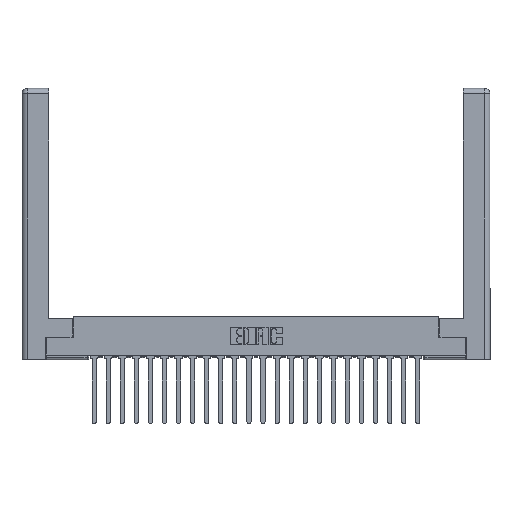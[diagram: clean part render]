
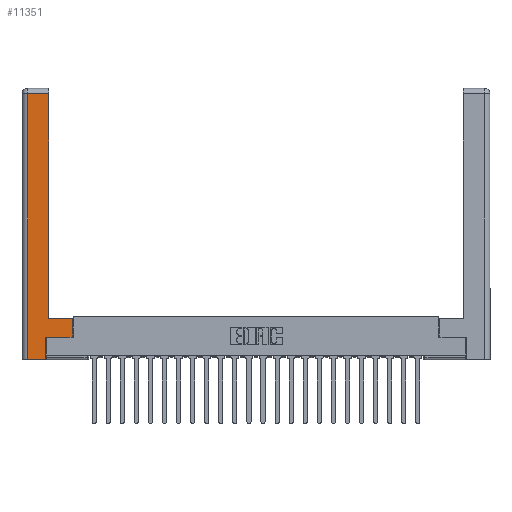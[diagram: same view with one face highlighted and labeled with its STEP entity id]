
A CAD part, top view. The second image highlights one B-rep face of the part: STEP entity #11351.
In plain terms, the highlighted planar face has unit normal (0, 0, 1).
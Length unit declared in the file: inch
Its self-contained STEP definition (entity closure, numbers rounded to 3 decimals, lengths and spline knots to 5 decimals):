
#398 = LINE ( 'NONE', #23268, #8163 ) ;
#634 = LINE ( 'NONE', #24262, #15480 ) ;
#1180 = ORIENTED_EDGE ( 'NONE', *, *, #20733, .T. ) ;
#2334 = CARTESIAN_POINT ( 'NONE',  ( 0.0615, 0., 0. ) ) ;
#2374 = EDGE_CURVE ( 'NONE', #14842, #12267, #24141, .T. ) ;
#2509 = CARTESIAN_POINT ( 'NONE',  ( 0.0615, 2.94, 0. ) ) ;
#2754 = DIRECTION ( 'NONE',  ( 0., 1., 0. ) ) ;
#2984 = CARTESIAN_POINT ( 'NONE',  ( 0.565, 0.45, 0. ) ) ;
#3222 = DIRECTION ( 'NONE',  ( -1., 0., 0. ) ) ;
#3646 = EDGE_CURVE ( 'NONE', #18784, #19529, #634, .T. ) ;
#4583 = CARTESIAN_POINT ( 'NONE',  ( 0.0615, 0., 0. ) ) ;
#5269 = CARTESIAN_POINT ( 'NONE',  ( 0.265, 0., 0. ) ) ;
#5600 = ORIENTED_EDGE ( 'NONE', *, *, #18948, .T. ) ;
#5623 = ORIENTED_EDGE ( 'NONE', *, *, #21719, .T. ) ;
#5715 = DIRECTION ( 'NONE',  ( -1., 0., 0. ) ) ;
#6089 = EDGE_CURVE ( 'NONE', #19529, #10679, #15363, .T. ) ;
#6569 = LINE ( 'NONE', #12348, #18218 ) ;
#6928 = VECTOR ( 'NONE', #14766, 39.37008 ) ;
#7038 = CARTESIAN_POINT ( 'NONE',  ( 0.295, 0.45, 0. ) ) ;
#7967 = CARTESIAN_POINT ( 'NONE',  ( 0.565, 0.245, 0. ) ) ;
#8163 = VECTOR ( 'NONE', #5715, 39.37008 ) ;
#8398 = DIRECTION ( 'NONE',  ( 0., -1., 0. ) ) ;
#8544 = ORIENTED_EDGE ( 'NONE', *, *, #2374, .T. ) ;
#9250 = CARTESIAN_POINT ( 'NONE',  ( 0.565, 0.245, 0. ) ) ;
#9595 = DIRECTION ( 'NONE',  ( 0., 1., 0. ) ) ;
#9754 = VERTEX_POINT ( 'NONE', #7967 ) ;
#10202 = ORIENTED_EDGE ( 'NONE', *, *, #23213, .T. ) ;
#10385 = AXIS2_PLACEMENT_3D ( 'NONE', #18745, #20805, #3222 ) ;
#10679 = VERTEX_POINT ( 'NONE', #16764 ) ;
#10880 = DIRECTION ( 'NONE',  ( 0., 1., 0. ) ) ;
#11351 = ADVANCED_FACE ( 'NONE', ( #16554 ), #14897, .F. ) ;
#11665 = ORIENTED_EDGE ( 'NONE', *, *, #3646, .T. ) ;
#11798 = VECTOR ( 'NONE', #2754, 39.37008 ) ;
#12267 = VERTEX_POINT ( 'NONE', #4583 ) ;
#12348 = CARTESIAN_POINT ( 'NONE',  ( 0.265, 0., 0. ) ) ;
#12502 = LINE ( 'NONE', #13232, #11798 ) ;
#13232 = CARTESIAN_POINT ( 'NONE',  ( 0.265, 0.245, 0. ) ) ;
#14766 = DIRECTION ( 'NONE',  ( 1., 0., 0. ) ) ;
#14842 = VERTEX_POINT ( 'NONE', #2509 ) ;
#14897 = PLANE ( 'NONE',  #10385 ) ;
#15363 = LINE ( 'NONE', #17395, #16961 ) ;
#15480 = VECTOR ( 'NONE', #18250, 39.37008 ) ;
#15583 = EDGE_LOOP ( 'NONE', ( #20561, #21468, #8544, #5600, #5623, #10202, #1180, #11665 ) ) ;
#15752 = CARTESIAN_POINT ( 'NONE',  ( 0.265, 0.245, 0. ) ) ;
#16011 = VERTEX_POINT ( 'NONE', #5269 ) ;
#16554 = FACE_OUTER_BOUND ( 'NONE', #15583, .T. ) ;
#16764 = CARTESIAN_POINT ( 'NONE',  ( 0.295, 2.94, 0. ) ) ;
#16961 = VECTOR ( 'NONE', #9595, 39.37008 ) ;
#17032 = CARTESIAN_POINT ( 'NONE',  ( 0.565, 0.45, 0. ) ) ;
#17395 = CARTESIAN_POINT ( 'NONE',  ( 0.295, 3., 0. ) ) ;
#18218 = VECTOR ( 'NONE', #18248, 39.37008 ) ;
#18248 = DIRECTION ( 'NONE',  ( 1., 0., 0. ) ) ;
#18250 = DIRECTION ( 'NONE',  ( -1., 0., 0. ) ) ;
#18745 = CARTESIAN_POINT ( 'NONE',  ( 0., 0., 0. ) ) ;
#18784 = VERTEX_POINT ( 'NONE', #2984 ) ;
#18846 = LINE ( 'NONE', #17032, #23189 ) ;
#18864 = LINE ( 'NONE', #9250, #6928 ) ;
#18948 = EDGE_CURVE ( 'NONE', #12267, #16011, #6569, .T. ) ;
#19529 = VERTEX_POINT ( 'NONE', #7038 ) ;
#20561 = ORIENTED_EDGE ( 'NONE', *, *, #6089, .T. ) ;
#20733 = EDGE_CURVE ( 'NONE', #9754, #18784, #18846, .T. ) ;
#20805 = DIRECTION ( 'NONE',  ( 0., 0., -1. ) ) ;
#20958 = VERTEX_POINT ( 'NONE', #15752 ) ;
#21468 = ORIENTED_EDGE ( 'NONE', *, *, #22585, .T. ) ;
#21719 = EDGE_CURVE ( 'NONE', #16011, #20958, #12502, .T. ) ;
#22585 = EDGE_CURVE ( 'NONE', #10679, #14842, #398, .T. ) ;
#23189 = VECTOR ( 'NONE', #10880, 39.37008 ) ;
#23213 = EDGE_CURVE ( 'NONE', #20958, #9754, #18864, .T. ) ;
#23268 = CARTESIAN_POINT ( 'NONE',  ( 0.0615, 2.94, 0. ) ) ;
#23620 = VECTOR ( 'NONE', #8398, 39.37008 ) ;
#24141 = LINE ( 'NONE', #2334, #23620 ) ;
#24262 = CARTESIAN_POINT ( 'NONE',  ( 0.295, 0.45, 0. ) ) ;
